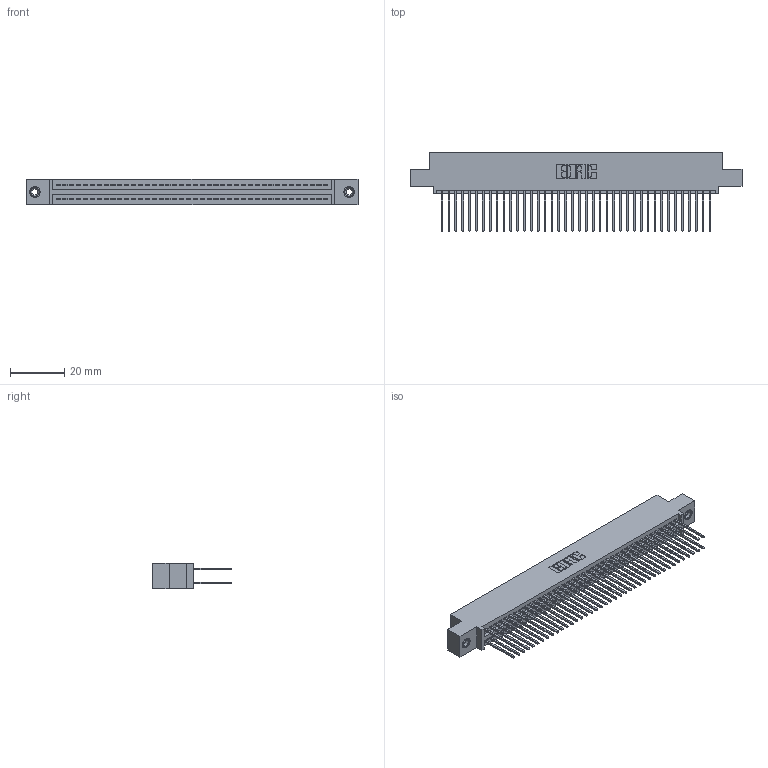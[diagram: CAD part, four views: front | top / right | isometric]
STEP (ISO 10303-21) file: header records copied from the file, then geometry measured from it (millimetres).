
FILE_DESCRIPTION (( 'STEP AP203' ), '1' );
FILE_NAME ('395-080-540-508.STEP', '2019-10-25T04:19:47', ( '' ), ( '' ), 'SwSTEP 2.0', 'SolidWorks 2016', '' );
FILE_SCHEMA (( 'CONFIG_CONTROL_DESIGN' ));
Length unit declared in the file: inch
Products named in the file (4): 345-292-001_345-293-140; 345-250-001_345-250-003-102; 395-080-540-508; 345 Part_0.110 Offset - 0.156 Dia-TI
Assembly tree (83 placements, depth 2):
  395-080-540-508
    345 Part_0.110 Offset - 0.156 Dia-TI
    345-292-001_345-293-140  x80
    345-250-001_345-250-003-102  x2
Bounding box: 122.81 x 29.13 x 9.4 mm (x, y, z)
Volume: 12134.6 mm3; surface area: 19411.6 mm2
Topology: 83 solids, 83 shells, 4190 faces, 12409 edges, 8158 vertices
Faces by surface type: plane 2756, cylinder 1418, cone 12, torus 4
Entity records: 32990 total; most frequent: CARTESIAN_POINT 5515, ORIENTED_EDGE 5442, DIRECTION 4891, EDGE_CURVE 2721, VECTOR 2409, LINE 2409, VERTEX_POINT 1808, AXIS2_PLACEMENT_3D 1241
